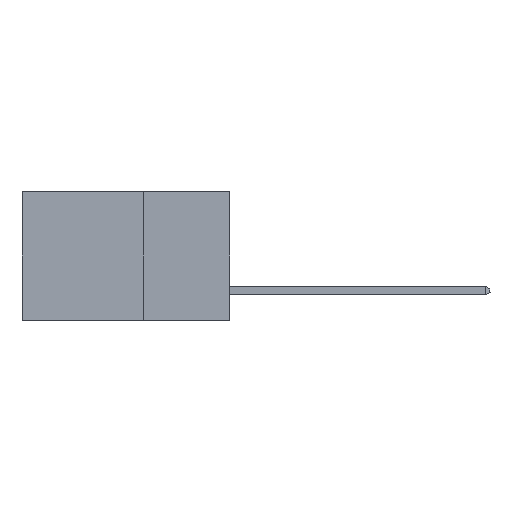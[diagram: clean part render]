
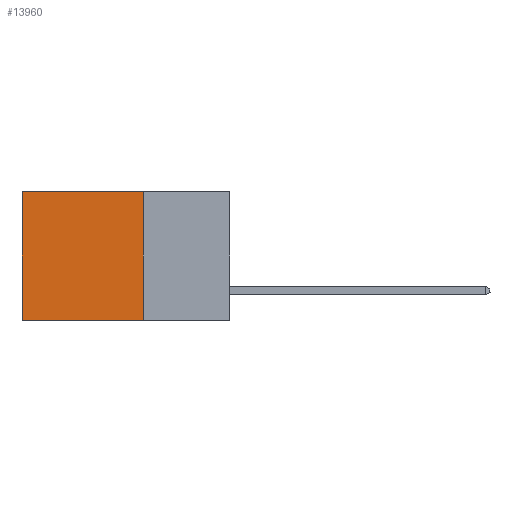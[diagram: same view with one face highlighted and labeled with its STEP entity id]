
A CAD part, left-side view. The second image highlights one B-rep face of the part: STEP entity #13960.
In plain terms, the highlighted planar face has unit normal (-1, 0, 0).
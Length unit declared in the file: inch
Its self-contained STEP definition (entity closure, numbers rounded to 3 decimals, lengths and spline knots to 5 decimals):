
#217 = CARTESIAN_POINT ( 'NONE',  ( 0.298, 0.25, 0. ) ) ;
#1367 = EDGE_CURVE ( 'NONE', #2726, #8656, #14484, .T. ) ;
#1606 = VECTOR ( 'NONE', #20234, 39.37008 ) ;
#2726 = VERTEX_POINT ( 'NONE', #16138 ) ;
#2744 = CARTESIAN_POINT ( 'NONE',  ( 0.298, 0.25, 0. ) ) ;
#5253 = EDGE_LOOP ( 'NONE', ( #22652, #5896, #10027, #15729 ) ) ;
#5263 = CARTESIAN_POINT ( 'NONE',  ( 0.298, 0.25, -0.37 ) ) ;
#5896 = ORIENTED_EDGE ( 'NONE', *, *, #10189, .F. ) ;
#6237 = CARTESIAN_POINT ( 'NONE',  ( 0.298, 0.6, -0.37 ) ) ;
#6344 = AXIS2_PLACEMENT_3D ( 'NONE', #217, #9285, #14826 ) ;
#6401 = VERTEX_POINT ( 'NONE', #6237 ) ;
#6636 = CARTESIAN_POINT ( 'NONE',  ( 0.298, 0.25, -0.37 ) ) ;
#7191 = VECTOR ( 'NONE', #9513, 39.37008 ) ;
#7491 = VERTEX_POINT ( 'NONE', #5263 ) ;
#8396 = CARTESIAN_POINT ( 'NONE',  ( 0.298, 0.25, 0. ) ) ;
#8656 = VERTEX_POINT ( 'NONE', #14590 ) ;
#9232 = VECTOR ( 'NONE', #12045, 39.37008 ) ;
#9285 = DIRECTION ( 'NONE',  ( 1., 0., 0. ) ) ;
#9513 = DIRECTION ( 'NONE',  ( 0., 0., -1. ) ) ;
#10027 = ORIENTED_EDGE ( 'NONE', *, *, #18185, .F. ) ;
#10189 = EDGE_CURVE ( 'NONE', #7491, #6401, #15895, .T. ) ;
#11908 = LINE ( 'NONE', #8396, #9232 ) ;
#12045 = DIRECTION ( 'NONE',  ( 0., 0., -1. ) ) ;
#13530 = FACE_OUTER_BOUND ( 'NONE', #5253, .T. ) ;
#13960 = ADVANCED_FACE ( 'NONE', ( #13530 ), #19973, .F. ) ;
#14484 = LINE ( 'NONE', #2744, #14765 ) ;
#14590 = CARTESIAN_POINT ( 'NONE',  ( 0.298, 0.6, 0. ) ) ;
#14765 = VECTOR ( 'NONE', #19126, 39.37008 ) ;
#14826 = DIRECTION ( 'NONE',  ( 0., 0., -1. ) ) ;
#15583 = EDGE_CURVE ( 'NONE', #8656, #6401, #16113, .T. ) ;
#15729 = ORIENTED_EDGE ( 'NONE', *, *, #1367, .T. ) ;
#15895 = LINE ( 'NONE', #6636, #1606 ) ;
#16113 = LINE ( 'NONE', #21916, #7191 ) ;
#16138 = CARTESIAN_POINT ( 'NONE',  ( 0.298, 0.25, 0. ) ) ;
#18185 = EDGE_CURVE ( 'NONE', #2726, #7491, #11908, .T. ) ;
#19126 = DIRECTION ( 'NONE',  ( 0., 1., 0. ) ) ;
#19973 = PLANE ( 'NONE',  #6344 ) ;
#20234 = DIRECTION ( 'NONE',  ( 0., 1., 0. ) ) ;
#21916 = CARTESIAN_POINT ( 'NONE',  ( 0.298, 0.6, 0. ) ) ;
#22652 = ORIENTED_EDGE ( 'NONE', *, *, #15583, .T. ) ;
